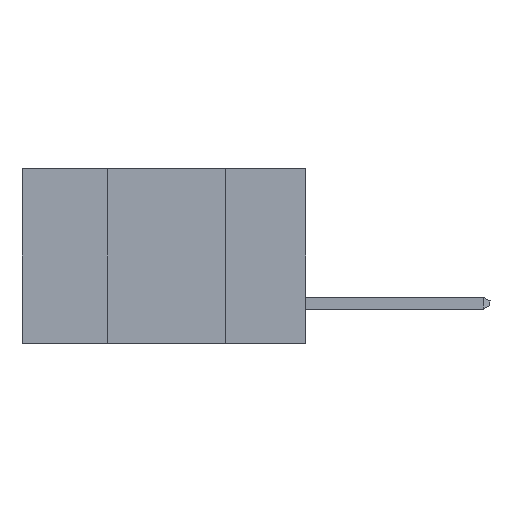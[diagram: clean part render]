
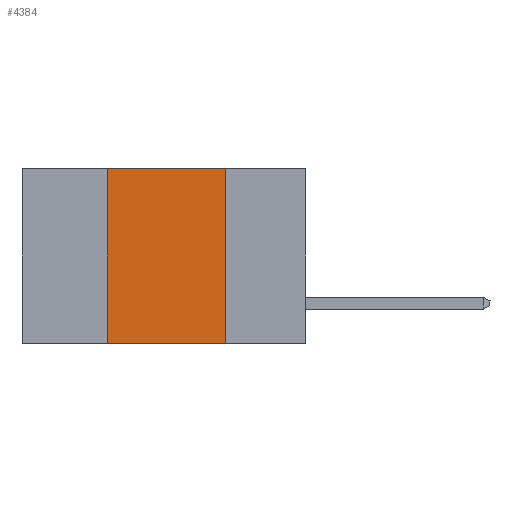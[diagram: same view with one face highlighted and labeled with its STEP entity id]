
A CAD part, left-side view. The second image highlights one B-rep face of the part: STEP entity #4384.
In plain terms, the highlighted planar face has unit normal (-1, 0, 0).
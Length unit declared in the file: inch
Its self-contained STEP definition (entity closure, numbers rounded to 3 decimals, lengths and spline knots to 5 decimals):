
#831 = LINE ( 'NONE', #10217, #4857 ) ;
#990 = CARTESIAN_POINT ( 'NONE',  ( 0., 0.17, 0. ) ) ;
#2299 = LINE ( 'NONE', #990, #11035 ) ;
#2769 = AXIS2_PLACEMENT_3D ( 'NONE', #6519, #9103, #9951 ) ;
#3329 = ORIENTED_EDGE ( 'NONE', *, *, #5373, .F. ) ;
#3431 = CARTESIAN_POINT ( 'NONE',  ( 0., 0.6, -0.37 ) ) ;
#4224 = ORIENTED_EDGE ( 'NONE', *, *, #4960, .F. ) ;
#4260 = VERTEX_POINT ( 'NONE', #6269 ) ;
#4276 = VERTEX_POINT ( 'NONE', #5386 ) ;
#4308 = CARTESIAN_POINT ( 'NONE',  ( 0., 0.6, 0. ) ) ;
#4384 = ADVANCED_FACE ( 'NONE', ( #8911 ), #8177, .F. ) ;
#4594 = LINE ( 'NONE', #4308, #5885 ) ;
#4857 = VECTOR ( 'NONE', #7781, 39.37008 ) ;
#4960 = EDGE_CURVE ( 'NONE', #4260, #6155, #2299, .T. ) ;
#5222 = LINE ( 'NONE', #3431, #5613 ) ;
#5373 = EDGE_CURVE ( 'NONE', #8561, #4260, #4594, .T. ) ;
#5380 = EDGE_CURVE ( 'NONE', #4276, #8561, #831, .T. ) ;
#5386 = CARTESIAN_POINT ( 'NONE',  ( 0., 0.42, -0.37 ) ) ;
#5613 = VECTOR ( 'NONE', #8236, 39.37008 ) ;
#5885 = VECTOR ( 'NONE', #9619, 39.37008 ) ;
#6155 = VERTEX_POINT ( 'NONE', #8135 ) ;
#6243 = ORIENTED_EDGE ( 'NONE', *, *, #8715, .T. ) ;
#6269 = CARTESIAN_POINT ( 'NONE',  ( 0., 0.17, 0. ) ) ;
#6519 = CARTESIAN_POINT ( 'NONE',  ( 0., 0.6, 0. ) ) ;
#7781 = DIRECTION ( 'NONE',  ( 0., 0., 1. ) ) ;
#8070 = EDGE_LOOP ( 'NONE', ( #4224, #3329, #8751, #6243 ) ) ;
#8135 = CARTESIAN_POINT ( 'NONE',  ( 0., 0.17, -0.37 ) ) ;
#8177 = PLANE ( 'NONE',  #2769 ) ;
#8236 = DIRECTION ( 'NONE',  ( 0., -1., 0. ) ) ;
#8561 = VERTEX_POINT ( 'NONE', #10439 ) ;
#8715 = EDGE_CURVE ( 'NONE', #4276, #6155, #5222, .T. ) ;
#8751 = ORIENTED_EDGE ( 'NONE', *, *, #5380, .F. ) ;
#8911 = FACE_OUTER_BOUND ( 'NONE', #8070, .T. ) ;
#9103 = DIRECTION ( 'NONE',  ( 1., 0., 0. ) ) ;
#9619 = DIRECTION ( 'NONE',  ( 0., -1., 0. ) ) ;
#9951 = DIRECTION ( 'NONE',  ( 0., 0., -1. ) ) ;
#10217 = CARTESIAN_POINT ( 'NONE',  ( 0., 0.42, 0. ) ) ;
#10356 = DIRECTION ( 'NONE',  ( 0., 0., -1. ) ) ;
#10439 = CARTESIAN_POINT ( 'NONE',  ( 0., 0.42, 0. ) ) ;
#11035 = VECTOR ( 'NONE', #10356, 39.37008 ) ;
